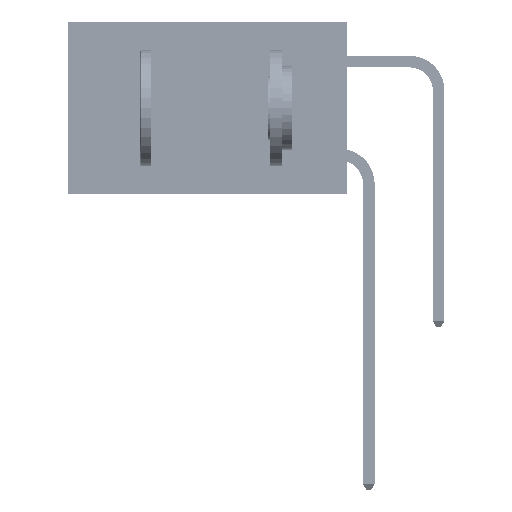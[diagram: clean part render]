
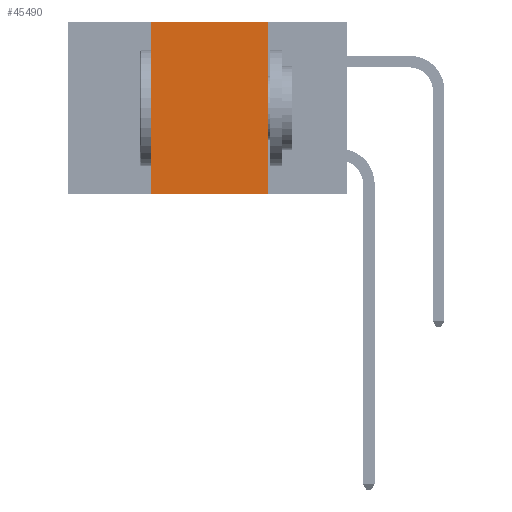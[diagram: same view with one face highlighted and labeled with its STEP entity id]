
A CAD part, left-side view. The second image highlights one B-rep face of the part: STEP entity #45490.
In plain terms, the highlighted planar face has unit normal (-1, 0, 0).
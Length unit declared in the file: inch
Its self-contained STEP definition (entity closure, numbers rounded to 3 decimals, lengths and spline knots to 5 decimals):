
#1918 = EDGE_CURVE ( 'NONE', #31838, #38553, #23475, .T. ) ;
#3306 = DIRECTION ( 'NONE',  ( 1., 0., 0. ) ) ;
#3965 = ORIENTED_EDGE ( 'NONE', *, *, #44767, .F. ) ;
#4324 = LINE ( 'NONE', #44196, #6767 ) ;
#4695 = CARTESIAN_POINT ( 'NONE',  ( 0., 0.6, -0.37 ) ) ;
#6572 = EDGE_CURVE ( 'NONE', #31838, #39336, #4324, .T. ) ;
#6767 = VECTOR ( 'NONE', #31939, 39.37008 ) ;
#7044 = CARTESIAN_POINT ( 'NONE',  ( 0., 0.42, 0. ) ) ;
#7243 = VECTOR ( 'NONE', #13836, 39.37008 ) ;
#7499 = ORIENTED_EDGE ( 'NONE', *, *, #1918, .T. ) ;
#12676 = VERTEX_POINT ( 'NONE', #32427 ) ;
#12992 = CARTESIAN_POINT ( 'NONE',  ( 0., 0.42, -0.37 ) ) ;
#13836 = DIRECTION ( 'NONE',  ( 0., 0., -1. ) ) ;
#14999 = CARTESIAN_POINT ( 'NONE',  ( 0., 0.17, -0.37 ) ) ;
#15324 = LINE ( 'NONE', #35993, #46785 ) ;
#15964 = ORIENTED_EDGE ( 'NONE', *, *, #6572, .F. ) ;
#16543 = DIRECTION ( 'NONE',  ( 0., -1., 0. ) ) ;
#19115 = PLANE ( 'NONE',  #38197 ) ;
#19285 = DIRECTION ( 'NONE',  ( 0., 0., -1. ) ) ;
#20167 = LINE ( 'NONE', #33464, #7243 ) ;
#23475 = LINE ( 'NONE', #4695, #24127 ) ;
#24127 = VECTOR ( 'NONE', #16543, 39.37008 ) ;
#31162 = EDGE_LOOP ( 'NONE', ( #3965, #33616, #15964, #7499 ) ) ;
#31838 = VERTEX_POINT ( 'NONE', #12992 ) ;
#31939 = DIRECTION ( 'NONE',  ( 0., 0., 1. ) ) ;
#32427 = CARTESIAN_POINT ( 'NONE',  ( 0., 0.17, 0. ) ) ;
#33464 = CARTESIAN_POINT ( 'NONE',  ( 0., 0.17, 0. ) ) ;
#33616 = ORIENTED_EDGE ( 'NONE', *, *, #33853, .F. ) ;
#33853 = EDGE_CURVE ( 'NONE', #39336, #12676, #15324, .T. ) ;
#35273 = CARTESIAN_POINT ( 'NONE',  ( 0., 0.6, 0. ) ) ;
#35812 = DIRECTION ( 'NONE',  ( 0., -1., 0. ) ) ;
#35993 = CARTESIAN_POINT ( 'NONE',  ( 0., 0.6, 0. ) ) ;
#38197 = AXIS2_PLACEMENT_3D ( 'NONE', #35273, #3306, #19285 ) ;
#38553 = VERTEX_POINT ( 'NONE', #14999 ) ;
#39336 = VERTEX_POINT ( 'NONE', #7044 ) ;
#44196 = CARTESIAN_POINT ( 'NONE',  ( 0., 0.42, 0. ) ) ;
#44767 = EDGE_CURVE ( 'NONE', #12676, #38553, #20167, .T. ) ;
#45490 = ADVANCED_FACE ( 'NONE', ( #49814 ), #19115, .F. ) ;
#46785 = VECTOR ( 'NONE', #35812, 39.37008 ) ;
#49814 = FACE_OUTER_BOUND ( 'NONE', #31162, .T. ) ;
